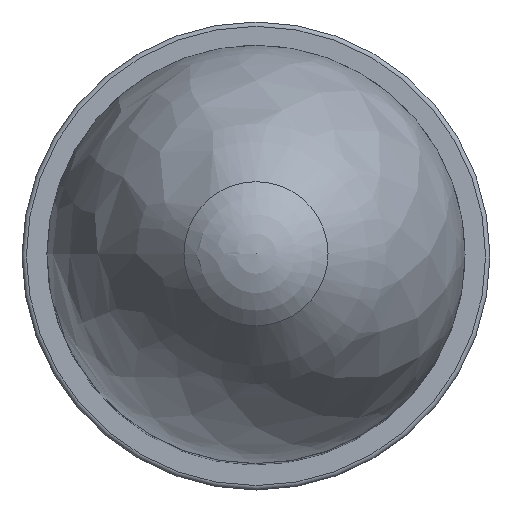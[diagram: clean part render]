
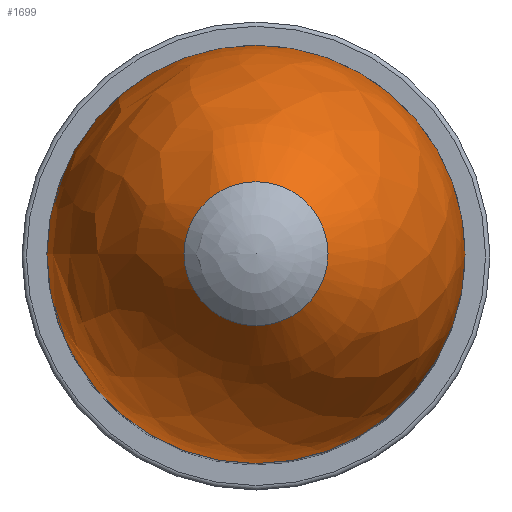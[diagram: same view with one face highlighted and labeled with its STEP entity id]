
A CAD part, top view. The second image highlights one B-rep face of the part: STEP entity #1699.
In plain terms, the highlighted free-form (B-spline) face has degree [2, 2] with [3, 9] control points.
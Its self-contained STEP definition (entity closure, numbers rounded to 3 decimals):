
#14=(
BOUNDED_SURFACE()
B_SPLINE_SURFACE(2,2,((#7469,#7470,#7471,#7472,#7473,#7474,#7475,#7476,
#7477),(#7478,#7479,#7480,#7481,#7482,#7483,#7484,#7485,#7486),(#7487,#7488,
#7489,#7490,#7491,#7492,#7493,#7494,#7495)),.UNSPECIFIED.,.F.,.T.,.F.)
B_SPLINE_SURFACE_WITH_KNOTS((3,3),(3,2,2,2,3),(0.,0.746),(-3.142,
-1.571,0.,1.571,3.142),.UNSPECIFIED.)
GEOMETRIC_REPRESENTATION_ITEM()
RATIONAL_B_SPLINE_SURFACE(((1.,0.707,1.,0.707,1.,
0.707,1.,0.707,1.),(0.931,0.658,
0.931,0.658,0.931,0.658,
0.931,0.658,0.931),(1.,0.707,
1.,0.707,1.,0.707,1.,0.707,1.)))
REPRESENTATION_ITEM('')
SURFACE()
);
#151=FACE_OUTER_BOUND('',#260,.T.);
#260=EDGE_LOOP('',(#1403,#1404,#1405,#1406,#1407));
#339=CIRCLE('',#1857,19.177);
#340=CIRCLE('',#1858,19.177);
#341=CIRCLE('',#1860,6.609);
#343=CIRCLE('',#1862,47.301);
#736=VERTEX_POINT('',#7459);
#737=VERTEX_POINT('',#7460);
#738=VERTEX_POINT('',#7465);
#966=EDGE_CURVE('',#736,#737,#339,.T.);
#968=EDGE_CURVE('',#737,#736,#340,.T.);
#969=EDGE_CURVE('',#738,#738,#341,.T.);
#971=EDGE_CURVE('',#738,#737,#343,.T.);
#1403=ORIENTED_EDGE('',*,*,#969,.F.);
#1404=ORIENTED_EDGE('',*,*,#971,.T.);
#1405=ORIENTED_EDGE('',*,*,#968,.T.);
#1406=ORIENTED_EDGE('',*,*,#966,.T.);
#1407=ORIENTED_EDGE('',*,*,#971,.F.);
#1699=ADVANCED_FACE('',(#151),#14,.F.);
#1857=AXIS2_PLACEMENT_3D('',#7461,#2155,#2156);
#1858=AXIS2_PLACEMENT_3D('',#7463,#2158,#2159);
#1860=AXIS2_PLACEMENT_3D('',#7466,#2162,#2163);
#1862=AXIS2_PLACEMENT_3D('',#7496,#2166,#2167);
#2155=DIRECTION('center_axis',(0.,0.,1.));
#2156=DIRECTION('ref_axis',(-1.,0.,0.));
#2158=DIRECTION('center_axis',(0.,0.,1.));
#2159=DIRECTION('ref_axis',(-1.,0.,0.));
#2162=DIRECTION('center_axis',(0.,0.,1.));
#2163=DIRECTION('ref_axis',(1.,0.,0.));
#2166=DIRECTION('center_axis',(0.,-1.,0.));
#2167=DIRECTION('ref_axis',(-1.,0.,0.));
#7459=CARTESIAN_POINT('',(19.177,0.,88.7));
#7460=CARTESIAN_POINT('',(-19.177,0.,88.7));
#7461=CARTESIAN_POINT('Origin',(0.,0.,88.7));
#7463=CARTESIAN_POINT('Origin',(0.,0.,88.7));
#7465=CARTESIAN_POINT('',(-6.609,0.,120.81));
#7466=CARTESIAN_POINT('Origin',(0.,0.,120.81));
#7469=CARTESIAN_POINT('Ctrl Pts',(-19.177,0.,88.7));
#7470=CARTESIAN_POINT('Ctrl Pts',(-19.177,-19.177,88.7));
#7471=CARTESIAN_POINT('Ctrl Pts',(0.,-19.177,88.7));
#7472=CARTESIAN_POINT('Ctrl Pts',(19.177,-19.177,88.7));
#7473=CARTESIAN_POINT('Ctrl Pts',(19.177,0.,88.7));
#7474=CARTESIAN_POINT('Ctrl Pts',(19.177,19.177,88.7));
#7475=CARTESIAN_POINT('Ctrl Pts',(0.,19.177,88.7));
#7476=CARTESIAN_POINT('Ctrl Pts',(-19.177,19.177,88.7));
#7477=CARTESIAN_POINT('Ctrl Pts',(-19.177,0.,88.7));
#7478=CARTESIAN_POINT('Ctrl Pts',(-19.177,0.,107.215));
#7479=CARTESIAN_POINT('Ctrl Pts',(-19.177,-19.177,107.215));
#7480=CARTESIAN_POINT('Ctrl Pts',(0.,-19.177,107.215));
#7481=CARTESIAN_POINT('Ctrl Pts',(19.177,-19.177,107.215));
#7482=CARTESIAN_POINT('Ctrl Pts',(19.177,0.,107.215));
#7483=CARTESIAN_POINT('Ctrl Pts',(19.177,19.177,107.215));
#7484=CARTESIAN_POINT('Ctrl Pts',(0.,19.177,107.215));
#7485=CARTESIAN_POINT('Ctrl Pts',(-19.177,19.177,107.215));
#7486=CARTESIAN_POINT('Ctrl Pts',(-19.177,0.,107.215));
#7487=CARTESIAN_POINT('Ctrl Pts',(-6.609,0.,120.81));
#7488=CARTESIAN_POINT('Ctrl Pts',(-6.609,-6.609,120.81));
#7489=CARTESIAN_POINT('Ctrl Pts',(0.,-6.609,
120.81));
#7490=CARTESIAN_POINT('Ctrl Pts',(6.609,-6.609,120.81));
#7491=CARTESIAN_POINT('Ctrl Pts',(6.609,0.,120.81));
#7492=CARTESIAN_POINT('Ctrl Pts',(6.609,6.609,120.81));
#7493=CARTESIAN_POINT('Ctrl Pts',(0.,6.609,
120.81));
#7494=CARTESIAN_POINT('Ctrl Pts',(-6.609,6.609,120.81));
#7495=CARTESIAN_POINT('Ctrl Pts',(-6.609,0.,120.81));
#7496=CARTESIAN_POINT('Origin',(28.124,0.,88.7));
